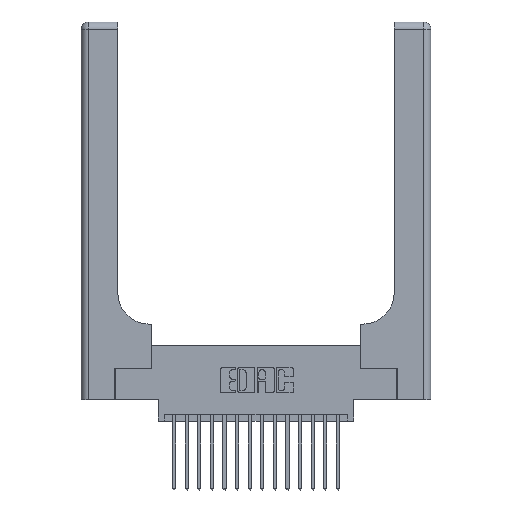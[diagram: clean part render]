
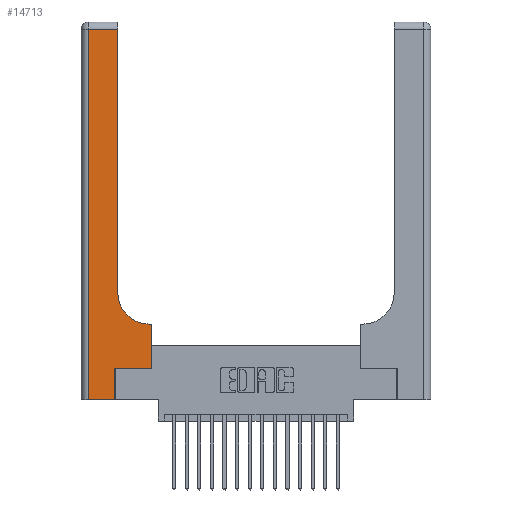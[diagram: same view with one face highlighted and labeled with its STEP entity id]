
A CAD part, top view. The second image highlights one B-rep face of the part: STEP entity #14713.
In plain terms, the highlighted planar face has unit normal (0, 0, 1).
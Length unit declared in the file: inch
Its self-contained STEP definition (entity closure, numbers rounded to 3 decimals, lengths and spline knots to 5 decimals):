
#736 = VERTEX_POINT ( 'NONE', #8704 ) ;
#933 = ORIENTED_EDGE ( 'NONE', *, *, #984, .T. ) ;
#984 = EDGE_CURVE ( 'NONE', #2455, #736, #6481, .T. ) ;
#1438 = CARTESIAN_POINT ( 'NONE',  ( 0.5585, 0.25, 0.37 ) ) ;
#1824 = LINE ( 'NONE', #19815, #2303 ) ;
#1982 = CARTESIAN_POINT ( 'NONE',  ( 0.06, 3., 0.37 ) ) ;
#2211 = CARTESIAN_POINT ( 'NONE',  ( 0.06, 2.94, 0.37 ) ) ;
#2303 = VECTOR ( 'NONE', #8990, 39.37008 ) ;
#2343 = VECTOR ( 'NONE', #5555, 39.37008 ) ;
#2455 = VERTEX_POINT ( 'NONE', #13175 ) ;
#2671 = EDGE_CURVE ( 'NONE', #16218, #16896, #1824, .T. ) ;
#3707 = VERTEX_POINT ( 'NONE', #6785 ) ;
#3821 = ORIENTED_EDGE ( 'NONE', *, *, #16377, .T. ) ;
#4028 = DIRECTION ( 'NONE',  ( 0., 1., 0. ) ) ;
#4356 = VECTOR ( 'NONE', #7536, 39.37008 ) ;
#4526 = CARTESIAN_POINT ( 'NONE',  ( 0., 3., 0.37 ) ) ;
#4565 = ORIENTED_EDGE ( 'NONE', *, *, #7904, .T. ) ;
#4814 = AXIS2_PLACEMENT_3D ( 'NONE', #4526, #15383, #6060 ) ;
#4849 = DIRECTION ( 'NONE',  ( -1., 0., 0. ) ) ;
#5130 = DIRECTION ( 'NONE',  ( 0., -1., 0. ) ) ;
#5333 = EDGE_CURVE ( 'NONE', #17274, #9581, #10214, .T. ) ;
#5555 = DIRECTION ( 'NONE',  ( 1., 0., 0. ) ) ;
#6060 = DIRECTION ( 'NONE',  ( -1., 0., 0. ) ) ;
#6161 = CARTESIAN_POINT ( 'NONE',  ( 0.269, 0.25, 0.37 ) ) ;
#6481 = LINE ( 'NONE', #6161, #2343 ) ;
#6730 = DIRECTION ( 'NONE',  ( 0., 0., -1. ) ) ;
#6785 = CARTESIAN_POINT ( 'NONE',  ( 0.5585, 0.6, 0.37 ) ) ;
#7536 = DIRECTION ( 'NONE',  ( 0., 1., 0. ) ) ;
#7646 = LINE ( 'NONE', #1438, #11786 ) ;
#7904 = EDGE_CURVE ( 'NONE', #16042, #16218, #14055, .T. ) ;
#7982 = LINE ( 'NONE', #9604, #19840 ) ;
#8403 = EDGE_CURVE ( 'NONE', #14023, #16042, #9875, .T. ) ;
#8441 = FACE_OUTER_BOUND ( 'NONE', #13268, .T. ) ;
#8704 = CARTESIAN_POINT ( 'NONE',  ( 0.5585, 0.25, 0.37 ) ) ;
#8779 = CARTESIAN_POINT ( 'NONE',  ( 0.06, 0., 0.37 ) ) ;
#8805 = ORIENTED_EDGE ( 'NONE', *, *, #8403, .T. ) ;
#8929 = LINE ( 'NONE', #9102, #4356 ) ;
#8990 = DIRECTION ( 'NONE',  ( 1., 0., 0. ) ) ;
#9102 = CARTESIAN_POINT ( 'NONE',  ( 0.269, 0., 0.37 ) ) ;
#9581 = VERTEX_POINT ( 'NONE', #10824 ) ;
#9604 = CARTESIAN_POINT ( 'NONE',  ( 0.2915, 0.6, 0.37 ) ) ;
#9875 = LINE ( 'NONE', #14142, #10361 ) ;
#9891 = VECTOR ( 'NONE', #5130, 39.37008 ) ;
#10214 = CIRCLE ( 'NONE', #12223, 0.25 ) ;
#10361 = VECTOR ( 'NONE', #4849, 39.37008 ) ;
#10824 = CARTESIAN_POINT ( 'NONE',  ( 0.2915, 0.85, 0.37 ) ) ;
#11661 = CARTESIAN_POINT ( 'NONE',  ( 0.2915, 2.94, 0.37 ) ) ;
#11738 = ORIENTED_EDGE ( 'NONE', *, *, #5333, .T. ) ;
#11755 = CARTESIAN_POINT ( 'NONE',  ( 0.2915, 3., 0.37 ) ) ;
#11786 = VECTOR ( 'NONE', #12330, 39.37008 ) ;
#11878 = ORIENTED_EDGE ( 'NONE', *, *, #14274, .T. ) ;
#12223 = AXIS2_PLACEMENT_3D ( 'NONE', #16057, #6730, #17616 ) ;
#12321 = ORIENTED_EDGE ( 'NONE', *, *, #14708, .T. ) ;
#12330 = DIRECTION ( 'NONE',  ( 0., 1., 0. ) ) ;
#13175 = CARTESIAN_POINT ( 'NONE',  ( 0.269, 0.25, 0.37 ) ) ;
#13268 = EDGE_LOOP ( 'NONE', ( #19997, #8805, #4565, #16102, #12321, #933, #3821, #11878, #11738 ) ) ;
#13374 = EDGE_CURVE ( 'NONE', #9581, #14023, #19609, .T. ) ;
#13825 = PLANE ( 'NONE',  #4814 ) ;
#14023 = VERTEX_POINT ( 'NONE', #11661 ) ;
#14055 = LINE ( 'NONE', #1982, #9891 ) ;
#14142 = CARTESIAN_POINT ( 'NONE',  ( 0., 2.94, 0.37 ) ) ;
#14274 = EDGE_CURVE ( 'NONE', #3707, #17274, #7982, .T. ) ;
#14708 = EDGE_CURVE ( 'NONE', #16896, #2455, #8929, .T. ) ;
#14713 = ADVANCED_FACE ( 'NONE', ( #8441 ), #13825, .F. ) ;
#15050 = VECTOR ( 'NONE', #4028, 39.37008 ) ;
#15315 = CARTESIAN_POINT ( 'NONE',  ( 0.269, 0., 0.37 ) ) ;
#15383 = DIRECTION ( 'NONE',  ( 0., 0., -1. ) ) ;
#16042 = VERTEX_POINT ( 'NONE', #2211 ) ;
#16057 = CARTESIAN_POINT ( 'NONE',  ( 0.5415, 0.85, 0.37 ) ) ;
#16102 = ORIENTED_EDGE ( 'NONE', *, *, #2671, .T. ) ;
#16218 = VERTEX_POINT ( 'NONE', #8779 ) ;
#16377 = EDGE_CURVE ( 'NONE', #736, #3707, #7646, .T. ) ;
#16896 = VERTEX_POINT ( 'NONE', #15315 ) ;
#17274 = VERTEX_POINT ( 'NONE', #17671 ) ;
#17616 = DIRECTION ( 'NONE',  ( 1., 0., 0. ) ) ;
#17671 = CARTESIAN_POINT ( 'NONE',  ( 0.5415, 0.6, 0.37 ) ) ;
#18914 = DIRECTION ( 'NONE',  ( -1., 0., 0. ) ) ;
#19609 = LINE ( 'NONE', #11755, #15050 ) ;
#19815 = CARTESIAN_POINT ( 'NONE',  ( 0., 0., 0.37 ) ) ;
#19840 = VECTOR ( 'NONE', #18914, 39.37008 ) ;
#19997 = ORIENTED_EDGE ( 'NONE', *, *, #13374, .T. ) ;
